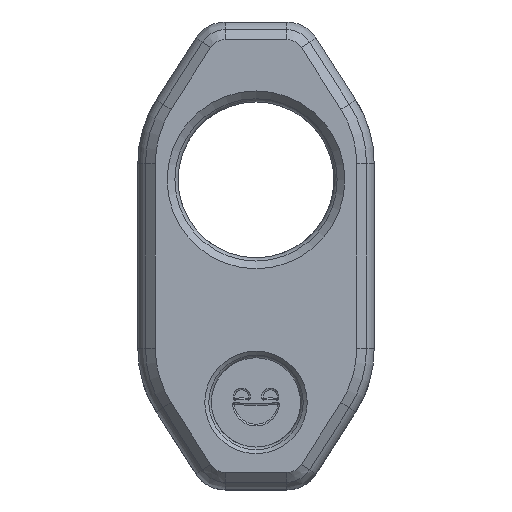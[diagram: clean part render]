
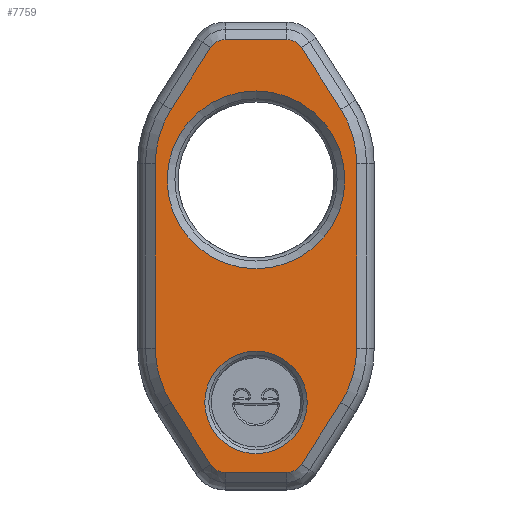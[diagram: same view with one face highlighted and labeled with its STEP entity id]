
A CAD part, front view. The second image highlights one B-rep face of the part: STEP entity #7759.
In plain terms, the highlighted planar face has unit normal (0, -1, 0).
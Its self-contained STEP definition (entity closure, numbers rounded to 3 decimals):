
#523=FACE_BOUND('',#2314,.T.);
#524=FACE_BOUND('',#2315,.T.);
#529=PLANE('',#8289);
#806=LINE('',#11275,#1294);
#807=LINE('',#11279,#1295);
#808=LINE('',#11283,#1296);
#809=LINE('',#11287,#1297);
#810=LINE('',#11291,#1298);
#811=LINE('',#11295,#1299);
#812=LINE('',#11299,#1300);
#813=LINE('',#11303,#1301);
#1294=VECTOR('',#9135,10.);
#1295=VECTOR('',#9138,10.);
#1296=VECTOR('',#9141,10.);
#1297=VECTOR('',#9144,10.);
#1298=VECTOR('',#9147,10.);
#1299=VECTOR('',#9150,10.);
#1300=VECTOR('',#9153,10.);
#1301=VECTOR('',#9156,10.);
#1806=FACE_OUTER_BOUND('',#2313,.T.);
#2313=EDGE_LOOP('',(#5235,#5236,#5237,#5238,#5239,#5240,#5241,#5242,#5243,
#5244,#5245,#5246,#5247,#5248,#5249,#5250));
#2314=EDGE_LOOP('',(#5251));
#2315=EDGE_LOOP('',(#5252));
#2828=CIRCLE('',#8284,10.15);
#2832=CIRCLE('',#8290,2.);
#2833=CIRCLE('',#8291,11.5);
#2834=CIRCLE('',#8292,11.5);
#2835=CIRCLE('',#8293,2.);
#2836=CIRCLE('',#8294,2.);
#2837=CIRCLE('',#8295,11.5);
#2838=CIRCLE('',#8296,11.5);
#2839=CIRCLE('',#8297,2.);
#2840=CIRCLE('',#8298,5.85);
#3234=VERTEX_POINT('',#11257);
#3240=VERTEX_POINT('',#11273);
#3241=VERTEX_POINT('',#11274);
#3242=VERTEX_POINT('',#11276);
#3243=VERTEX_POINT('',#11278);
#3244=VERTEX_POINT('',#11280);
#3245=VERTEX_POINT('',#11282);
#3246=VERTEX_POINT('',#11284);
#3247=VERTEX_POINT('',#11286);
#3248=VERTEX_POINT('',#11288);
#3249=VERTEX_POINT('',#11290);
#3250=VERTEX_POINT('',#11292);
#3251=VERTEX_POINT('',#11294);
#3252=VERTEX_POINT('',#11296);
#3253=VERTEX_POINT('',#11298);
#3254=VERTEX_POINT('',#11300);
#3255=VERTEX_POINT('',#11302);
#3256=VERTEX_POINT('',#11305);
#3975=EDGE_CURVE('',#3234,#3234,#2828,.T.);
#3983=EDGE_CURVE('',#3240,#3241,#806,.T.);
#3984=EDGE_CURVE('',#3240,#3242,#2832,.T.);
#3985=EDGE_CURVE('',#3242,#3243,#807,.T.);
#3986=EDGE_CURVE('',#3243,#3244,#2833,.T.);
#3987=EDGE_CURVE('',#3244,#3245,#808,.T.);
#3988=EDGE_CURVE('',#3245,#3246,#2834,.T.);
#3989=EDGE_CURVE('',#3246,#3247,#809,.T.);
#3990=EDGE_CURVE('',#3247,#3248,#2835,.T.);
#3991=EDGE_CURVE('',#3248,#3249,#810,.T.);
#3992=EDGE_CURVE('',#3250,#3249,#2836,.T.);
#3993=EDGE_CURVE('',#3251,#3250,#811,.T.);
#3994=EDGE_CURVE('',#3252,#3251,#2837,.T.);
#3995=EDGE_CURVE('',#3253,#3252,#812,.T.);
#3996=EDGE_CURVE('',#3254,#3253,#2838,.T.);
#3997=EDGE_CURVE('',#3255,#3254,#813,.T.);
#3998=EDGE_CURVE('',#3241,#3255,#2839,.T.);
#3999=EDGE_CURVE('',#3256,#3256,#2840,.T.);
#5235=ORIENTED_EDGE('',*,*,#3983,.F.);
#5236=ORIENTED_EDGE('',*,*,#3984,.T.);
#5237=ORIENTED_EDGE('',*,*,#3985,.T.);
#5238=ORIENTED_EDGE('',*,*,#3986,.T.);
#5239=ORIENTED_EDGE('',*,*,#3987,.T.);
#5240=ORIENTED_EDGE('',*,*,#3988,.T.);
#5241=ORIENTED_EDGE('',*,*,#3989,.T.);
#5242=ORIENTED_EDGE('',*,*,#3990,.T.);
#5243=ORIENTED_EDGE('',*,*,#3991,.T.);
#5244=ORIENTED_EDGE('',*,*,#3992,.F.);
#5245=ORIENTED_EDGE('',*,*,#3993,.F.);
#5246=ORIENTED_EDGE('',*,*,#3994,.F.);
#5247=ORIENTED_EDGE('',*,*,#3995,.F.);
#5248=ORIENTED_EDGE('',*,*,#3996,.F.);
#5249=ORIENTED_EDGE('',*,*,#3997,.F.);
#5250=ORIENTED_EDGE('',*,*,#3998,.F.);
#5251=ORIENTED_EDGE('',*,*,#3999,.T.);
#5252=ORIENTED_EDGE('',*,*,#3975,.F.);
#7759=ADVANCED_FACE('',(#1806,#523,#524),#529,.T.);
#8284=AXIS2_PLACEMENT_3D('',#11258,#9119,#9120);
#8289=AXIS2_PLACEMENT_3D('',#11272,#9133,#9134);
#8290=AXIS2_PLACEMENT_3D('',#11277,#9136,#9137);
#8291=AXIS2_PLACEMENT_3D('',#11281,#9139,#9140);
#8292=AXIS2_PLACEMENT_3D('',#11285,#9142,#9143);
#8293=AXIS2_PLACEMENT_3D('',#11289,#9145,#9146);
#8294=AXIS2_PLACEMENT_3D('',#11293,#9148,#9149);
#8295=AXIS2_PLACEMENT_3D('',#11297,#9151,#9152);
#8296=AXIS2_PLACEMENT_3D('',#11301,#9154,#9155);
#8297=AXIS2_PLACEMENT_3D('',#11304,#9157,#9158);
#8298=AXIS2_PLACEMENT_3D('',#11306,#9159,#9160);
#9119=DIRECTION('center_axis',(0.,-1.,0.));
#9120=DIRECTION('ref_axis',(1.,0.,0.));
#9133=DIRECTION('center_axis',(0.,-1.,0.));
#9134=DIRECTION('ref_axis',(1.,0.,0.));
#9135=DIRECTION('',(1.,0.,0.));
#9136=DIRECTION('center_axis',(0.,-1.,0.));
#9137=DIRECTION('ref_axis',(-0.481,0.,0.877));
#9138=DIRECTION('',(-0.538,0.,-0.843));
#9139=DIRECTION('center_axis',(0.,-1.,0.));
#9140=DIRECTION('ref_axis',(-0.96,0.,0.28));
#9141=DIRECTION('',(0.,0.,-1.));
#9142=DIRECTION('center_axis',(0.,-1.,0.));
#9143=DIRECTION('ref_axis',(-0.96,0.,-0.28));
#9144=DIRECTION('',(0.538,0.,-0.843));
#9145=DIRECTION('center_axis',(0.,-1.,0.));
#9146=DIRECTION('ref_axis',(-0.481,0.,-0.877));
#9147=DIRECTION('',(1.,0.,0.));
#9148=DIRECTION('center_axis',(0.,1.,0.));
#9149=DIRECTION('ref_axis',(0.481,0.,-0.877));
#9150=DIRECTION('',(-0.538,0.,-0.843));
#9151=DIRECTION('center_axis',(0.,1.,0.));
#9152=DIRECTION('ref_axis',(0.96,0.,-0.28));
#9153=DIRECTION('',(0.,0.,-1.));
#9154=DIRECTION('center_axis',(0.,1.,0.));
#9155=DIRECTION('ref_axis',(0.96,0.,0.28));
#9156=DIRECTION('',(0.538,0.,-0.843));
#9157=DIRECTION('center_axis',(0.,1.,0.));
#9158=DIRECTION('ref_axis',(0.481,0.,0.877));
#9159=DIRECTION('center_axis',(0.,1.,0.));
#9160=DIRECTION('ref_axis',(-1.,0.,0.));
#11257=CARTESIAN_POINT('',(-10.15,164.049,126.419));
#11258=CARTESIAN_POINT('Origin',(0.,164.049,
126.419));
#11272=CARTESIAN_POINT('Origin',(0.,164.049,
126.419));
#11273=CARTESIAN_POINT('',(-3.508,164.049,142.449));
#11274=CARTESIAN_POINT('',(3.508,164.049,142.449));
#11275=CARTESIAN_POINT('',(-2.258,164.049,142.449));
#11276=CARTESIAN_POINT('',(-5.195,164.049,141.524));
#11277=CARTESIAN_POINT('Origin',(-3.508,164.049,140.449));
#11278=CARTESIAN_POINT('',(-9.697,164.049,134.461));
#11279=CARTESIAN_POINT('',(-7.107,164.049,138.525));
#11280=CARTESIAN_POINT('',(-11.5,164.049,128.28));
#11281=CARTESIAN_POINT('Origin',(0.,164.049,
128.28));
#11282=CARTESIAN_POINT('',(-11.5,164.049,107.17));
#11283=CARTESIAN_POINT('',(-11.5,164.049,126.419));
#11284=CARTESIAN_POINT('',(-9.697,164.049,100.988));
#11285=CARTESIAN_POINT('Origin',(0.,164.049,
107.17));
#11286=CARTESIAN_POINT('',(-5.195,164.049,93.925));
#11287=CARTESIAN_POINT('',(-11.048,164.049,103.106));
#11288=CARTESIAN_POINT('',(-3.508,164.049,93.));
#11289=CARTESIAN_POINT('Origin',(-3.508,164.049,95.));
#11290=CARTESIAN_POINT('',(3.508,164.049,93.));
#11291=CARTESIAN_POINT('',(-6.75,164.049,93.));
#11292=CARTESIAN_POINT('',(5.195,164.049,93.925));
#11293=CARTESIAN_POINT('Origin',(3.508,164.049,95.));
#11294=CARTESIAN_POINT('',(9.697,164.049,100.988));
#11295=CARTESIAN_POINT('',(11.048,164.049,103.106));
#11296=CARTESIAN_POINT('',(11.5,164.049,107.17));
#11297=CARTESIAN_POINT('Origin',(0.,164.049,
107.17));
#11298=CARTESIAN_POINT('',(11.5,164.049,128.28));
#11299=CARTESIAN_POINT('',(11.5,164.049,126.419));
#11300=CARTESIAN_POINT('',(9.697,164.049,134.461));
#11301=CARTESIAN_POINT('Origin',(0.,164.049,
128.28));
#11302=CARTESIAN_POINT('',(5.195,164.049,141.524));
#11303=CARTESIAN_POINT('',(7.107,164.049,138.525));
#11304=CARTESIAN_POINT('Origin',(3.508,164.049,140.449));
#11305=CARTESIAN_POINT('',(-5.85,164.049,101.));
#11306=CARTESIAN_POINT('Origin',(0.,164.049,
101.));
